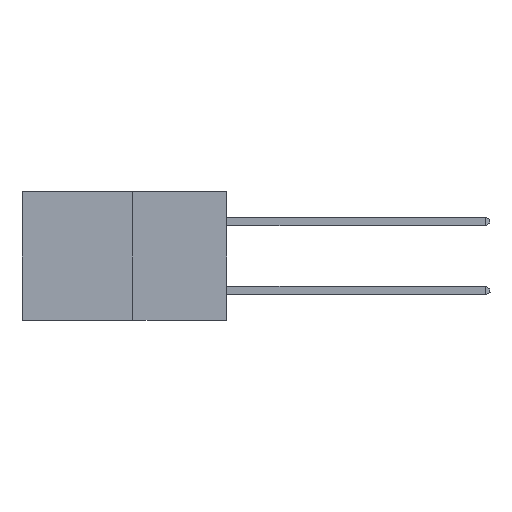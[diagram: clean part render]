
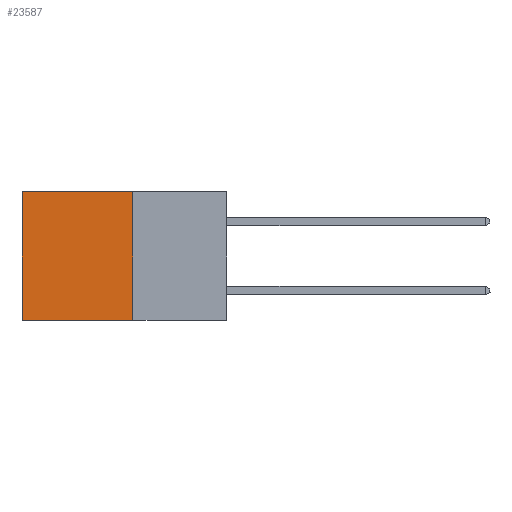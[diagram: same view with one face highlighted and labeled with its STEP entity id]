
A CAD part, left-side view. The second image highlights one B-rep face of the part: STEP entity #23587.
In plain terms, the highlighted planar face has unit normal (-1, 0, 0).
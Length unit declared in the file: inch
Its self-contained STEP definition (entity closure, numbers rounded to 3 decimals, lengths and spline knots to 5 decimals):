
#2521 = CARTESIAN_POINT ( 'NONE',  ( 0.277, 0.59, -0.37 ) ) ;
#2763 = CARTESIAN_POINT ( 'NONE',  ( 0.277, 0.59, -0.37 ) ) ;
#3026 = CARTESIAN_POINT ( 'NONE',  ( 0.277, 0.59, 0. ) ) ;
#4032 = CARTESIAN_POINT ( 'NONE',  ( 0.277, 0.27, 0. ) ) ;
#5991 = PLANE ( 'NONE',  #17351 ) ;
#6064 = LINE ( 'NONE', #11296, #16443 ) ;
#6465 = VERTEX_POINT ( 'NONE', #2763 ) ;
#6627 = VECTOR ( 'NONE', #14955, 39.37008 ) ;
#7265 = ORIENTED_EDGE ( 'NONE', *, *, #20660, .F. ) ;
#7522 = EDGE_LOOP ( 'NONE', ( #10609, #7265, #22921, #22256 ) ) ;
#8071 = DIRECTION ( 'NONE',  ( 1., 0., 0. ) ) ;
#8261 = CARTESIAN_POINT ( 'NONE',  ( 0.277, 0.27, 0. ) ) ;
#8280 = VERTEX_POINT ( 'NONE', #4032 ) ;
#8902 = VECTOR ( 'NONE', #9350, 39.37008 ) ;
#9274 = EDGE_CURVE ( 'NONE', #8280, #16872, #10858, .T. ) ;
#9350 = DIRECTION ( 'NONE',  ( 0., 0., -1. ) ) ;
#10609 = ORIENTED_EDGE ( 'NONE', *, *, #18276, .T. ) ;
#10858 = LINE ( 'NONE', #19610, #8902 ) ;
#11296 = CARTESIAN_POINT ( 'NONE',  ( 0.277, 0.27, -0.37 ) ) ;
#11471 = FACE_OUTER_BOUND ( 'NONE', #7522, .T. ) ;
#12139 = LINE ( 'NONE', #2521, #6627 ) ;
#13387 = DIRECTION ( 'NONE',  ( 0., 1., 0. ) ) ;
#14955 = DIRECTION ( 'NONE',  ( 0., 0., -1. ) ) ;
#15239 = LINE ( 'NONE', #8261, #19380 ) ;
#16176 = VERTEX_POINT ( 'NONE', #3026 ) ;
#16443 = VECTOR ( 'NONE', #13387, 39.37008 ) ;
#16872 = VERTEX_POINT ( 'NONE', #19017 ) ;
#17351 = AXIS2_PLACEMENT_3D ( 'NONE', #20384, #8071, #22437 ) ;
#18276 = EDGE_CURVE ( 'NONE', #16176, #6465, #12139, .T. ) ;
#19017 = CARTESIAN_POINT ( 'NONE',  ( 0.277, 0.27, -0.37 ) ) ;
#19380 = VECTOR ( 'NONE', #24514, 39.37008 ) ;
#19610 = CARTESIAN_POINT ( 'NONE',  ( 0.277, 0.27, -0.37 ) ) ;
#20384 = CARTESIAN_POINT ( 'NONE',  ( 0.277, 0.27, -0.37 ) ) ;
#20660 = EDGE_CURVE ( 'NONE', #16872, #6465, #6064, .T. ) ;
#22256 = ORIENTED_EDGE ( 'NONE', *, *, #25721, .T. ) ;
#22437 = DIRECTION ( 'NONE',  ( 0., 0., -1. ) ) ;
#22921 = ORIENTED_EDGE ( 'NONE', *, *, #9274, .F. ) ;
#23587 = ADVANCED_FACE ( 'NONE', ( #11471 ), #5991, .F. ) ;
#24514 = DIRECTION ( 'NONE',  ( 0., 1., 0. ) ) ;
#25721 = EDGE_CURVE ( 'NONE', #8280, #16176, #15239, .T. ) ;
